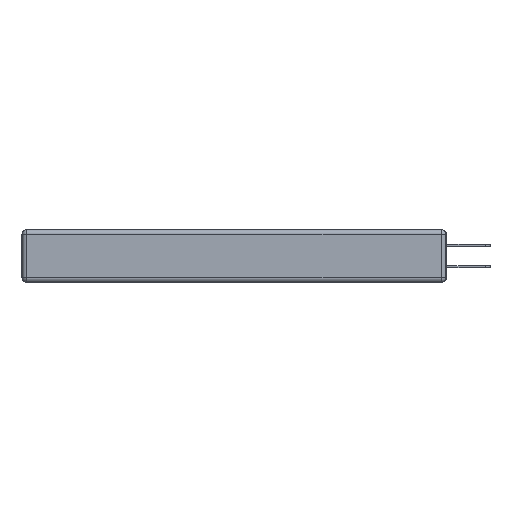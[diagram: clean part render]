
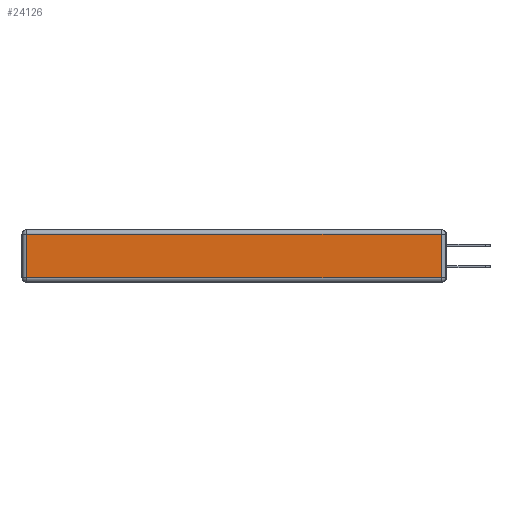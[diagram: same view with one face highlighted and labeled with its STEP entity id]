
A CAD part, left-side view. The second image highlights one B-rep face of the part: STEP entity #24126.
In plain terms, the highlighted planar face has unit normal (-1, 0, 0).
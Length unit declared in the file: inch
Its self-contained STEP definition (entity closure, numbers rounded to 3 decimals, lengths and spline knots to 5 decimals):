
#820 = CARTESIAN_POINT ( 'NONE',  ( 0., 2.72, -0.313 ) ) ;
#1255 = PLANE ( 'NONE',  #5549 ) ;
#1565 = CARTESIAN_POINT ( 'NONE',  ( 0., 2.72, -0.03 ) ) ;
#1888 = LINE ( 'NONE', #27211, #16147 ) ;
#1950 = CARTESIAN_POINT ( 'NONE',  ( 0., 2.72, -0.343 ) ) ;
#2078 = LINE ( 'NONE', #2672, #5879 ) ;
#2672 = CARTESIAN_POINT ( 'NONE',  ( 0., 2.75, -0.03 ) ) ;
#2714 = EDGE_CURVE ( 'NONE', #16620, #8929, #1888, .T. ) ;
#3473 = VERTEX_POINT ( 'NONE', #1565 ) ;
#5549 = AXIS2_PLACEMENT_3D ( 'NONE', #6210, #13500, #27874 ) ;
#5879 = VECTOR ( 'NONE', #16919, 39.37008 ) ;
#6210 = CARTESIAN_POINT ( 'NONE',  ( 0., 0., -0.343 ) ) ;
#6721 = VECTOR ( 'NONE', #14131, 39.37008 ) ;
#6938 = CARTESIAN_POINT ( 'NONE',  ( 0., 0., -0.313 ) ) ;
#8531 = DIRECTION ( 'NONE',  ( 0., 0., 1. ) ) ;
#8929 = VERTEX_POINT ( 'NONE', #15264 ) ;
#9335 = ORIENTED_EDGE ( 'NONE', *, *, #23238, .T. ) ;
#13315 = ORIENTED_EDGE ( 'NONE', *, *, #14608, .T. ) ;
#13500 = DIRECTION ( 'NONE',  ( -1., 0., 0. ) ) ;
#14131 = DIRECTION ( 'NONE',  ( 0., -1., 0. ) ) ;
#14608 = EDGE_CURVE ( 'NONE', #19583, #16620, #16791, .T. ) ;
#15264 = CARTESIAN_POINT ( 'NONE',  ( 0., 0.03, -0.03 ) ) ;
#15884 = FACE_OUTER_BOUND ( 'NONE', #25622, .T. ) ;
#16147 = VECTOR ( 'NONE', #8531, 39.37008 ) ;
#16620 = VERTEX_POINT ( 'NONE', #26103 ) ;
#16791 = LINE ( 'NONE', #6938, #6721 ) ;
#16901 = VECTOR ( 'NONE', #30476, 39.37008 ) ;
#16919 = DIRECTION ( 'NONE',  ( 0., 1., 0. ) ) ;
#19583 = VERTEX_POINT ( 'NONE', #820 ) ;
#22015 = ORIENTED_EDGE ( 'NONE', *, *, #2714, .T. ) ;
#23238 = EDGE_CURVE ( 'NONE', #8929, #3473, #2078, .T. ) ;
#24126 = ADVANCED_FACE ( 'NONE', ( #15884 ), #1255, .T. ) ;
#24156 = ORIENTED_EDGE ( 'NONE', *, *, #29648, .T. ) ;
#25622 = EDGE_LOOP ( 'NONE', ( #13315, #22015, #9335, #24156 ) ) ;
#26103 = CARTESIAN_POINT ( 'NONE',  ( 0., 0.03, -0.313 ) ) ;
#26566 = LINE ( 'NONE', #1950, #16901 ) ;
#27211 = CARTESIAN_POINT ( 'NONE',  ( 0., 0.03, -0.343 ) ) ;
#27874 = DIRECTION ( 'NONE',  ( 0., 0., 1. ) ) ;
#29648 = EDGE_CURVE ( 'NONE', #3473, #19583, #26566, .T. ) ;
#30476 = DIRECTION ( 'NONE',  ( 0., 0., -1. ) ) ;
